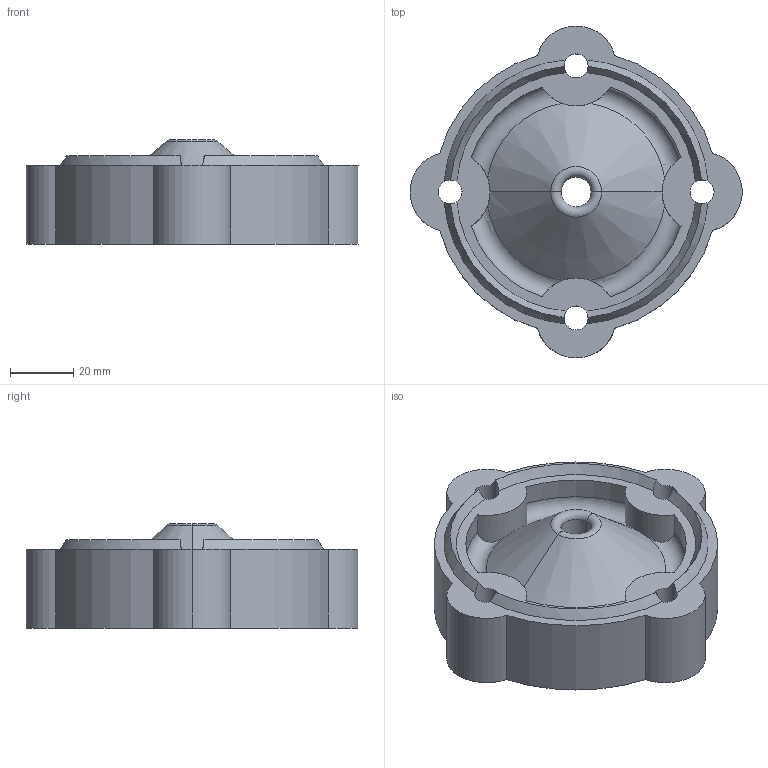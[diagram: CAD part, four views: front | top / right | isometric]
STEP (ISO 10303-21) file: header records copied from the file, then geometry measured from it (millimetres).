
FILE_DESCRIPTION (( 'STEP AP214' ), '1' );
FILE_NAME ('Cap.STEP', '2020-09-22T17:13:03', ( '' ), ( '' ), 'SwSTEP 2.0', 'SolidWorks 2019', '' );
FILE_SCHEMA (( 'AUTOMOTIVE_DESIGN' ));
Length unit declared in the file: millimetre
Products named in the file (1): Cap
Bounding box: 105.35 x 105.3 x 33.09 mm (x, y, z)
Volume: 155141.7 mm3; surface area: 28255.1 mm2
Topology: 1 solids, 1 shells, 47 faces, 139 edges, 91 vertices
Faces by surface type: cylinder 28, cone 10, torus 6, plane 3
Entity records: 1932 total; most frequent: CARTESIAN_POINT 616, ORIENTED_EDGE 278, DIRECTION 276, EDGE_CURVE 139, AXIS2_PLACEMENT_3D 123, VERTEX_POINT 91, CIRCLE 75, EDGE_LOOP 54
